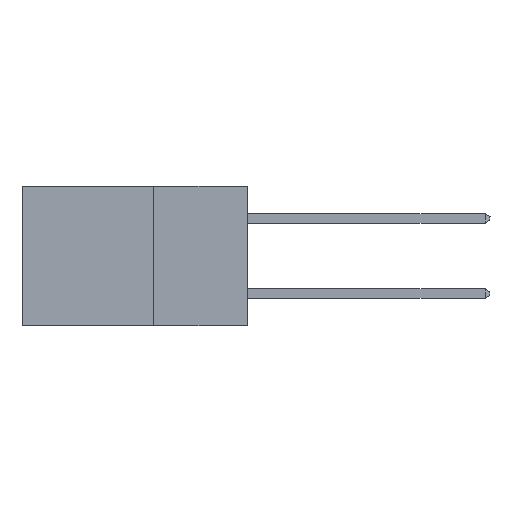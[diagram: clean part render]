
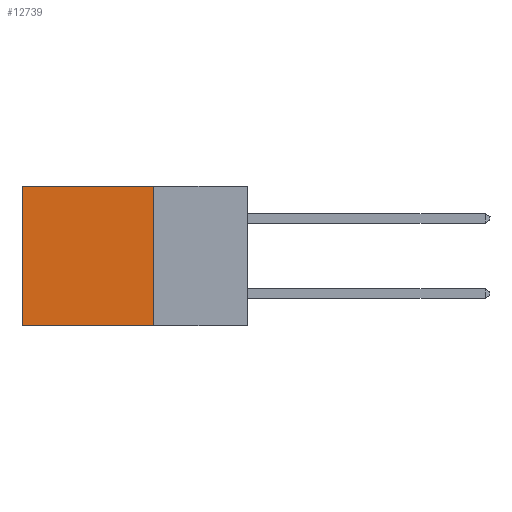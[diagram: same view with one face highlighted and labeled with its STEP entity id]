
A CAD part, left-side view. The second image highlights one B-rep face of the part: STEP entity #12739.
In plain terms, the highlighted planar face has unit normal (-1, 0, 0).
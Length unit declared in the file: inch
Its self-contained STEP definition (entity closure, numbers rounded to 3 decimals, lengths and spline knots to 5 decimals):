
#1129 = LINE ( 'NONE', #12004, #6805 ) ;
#2747 = CARTESIAN_POINT ( 'NONE',  ( 0.298, 0.25, -0.37 ) ) ;
#2850 = CARTESIAN_POINT ( 'NONE',  ( 0.298, 0.25, 0. ) ) ;
#3211 = LINE ( 'NONE', #12573, #20310 ) ;
#3948 = VECTOR ( 'NONE', #9587, 39.37008 ) ;
#4928 = DIRECTION ( 'NONE',  ( 0., 0., -1. ) ) ;
#5173 = VERTEX_POINT ( 'NONE', #20857 ) ;
#6610 = CARTESIAN_POINT ( 'NONE',  ( 0.298, 0.25, 0. ) ) ;
#6683 = DIRECTION ( 'NONE',  ( 1., 0., 0. ) ) ;
#6805 = VECTOR ( 'NONE', #4928, 39.37008 ) ;
#7255 = VERTEX_POINT ( 'NONE', #2850 ) ;
#7621 = EDGE_CURVE ( 'NONE', #7255, #5173, #3211, .T. ) ;
#7803 = FACE_OUTER_BOUND ( 'NONE', #18617, .T. ) ;
#9323 = EDGE_CURVE ( 'NONE', #5173, #23420, #1129, .T. ) ;
#9587 = DIRECTION ( 'NONE',  ( 0., 1., 0. ) ) ;
#10266 = DIRECTION ( 'NONE',  ( 0., 0., -1. ) ) ;
#10966 = ORIENTED_EDGE ( 'NONE', *, *, #9323, .T. ) ;
#11480 = VECTOR ( 'NONE', #19633, 39.37008 ) ;
#12004 = CARTESIAN_POINT ( 'NONE',  ( 0.298, 0.6, 0. ) ) ;
#12305 = CARTESIAN_POINT ( 'NONE',  ( 0.298, 0.25, 0. ) ) ;
#12573 = CARTESIAN_POINT ( 'NONE',  ( 0.298, 0.25, 0. ) ) ;
#12739 = ADVANCED_FACE ( 'NONE', ( #7803 ), #17516, .F. ) ;
#14529 = ORIENTED_EDGE ( 'NONE', *, *, #22888, .F. ) ;
#15287 = CARTESIAN_POINT ( 'NONE',  ( 0.298, 0.6, -0.37 ) ) ;
#16103 = ORIENTED_EDGE ( 'NONE', *, *, #18044, .F. ) ;
#16333 = LINE ( 'NONE', #12305, #11480 ) ;
#16691 = VERTEX_POINT ( 'NONE', #2747 ) ;
#16697 = ORIENTED_EDGE ( 'NONE', *, *, #7621, .T. ) ;
#17516 = PLANE ( 'NONE',  #18256 ) ;
#18044 = EDGE_CURVE ( 'NONE', #7255, #16691, #16333, .T. ) ;
#18256 = AXIS2_PLACEMENT_3D ( 'NONE', #6610, #6683, #10266 ) ;
#18617 = EDGE_LOOP ( 'NONE', ( #10966, #14529, #16103, #16697 ) ) ;
#18750 = CARTESIAN_POINT ( 'NONE',  ( 0.298, 0.25, -0.37 ) ) ;
#19633 = DIRECTION ( 'NONE',  ( 0., 0., -1. ) ) ;
#19653 = DIRECTION ( 'NONE',  ( 0., 1., 0. ) ) ;
#20225 = LINE ( 'NONE', #18750, #3948 ) ;
#20310 = VECTOR ( 'NONE', #19653, 39.37008 ) ;
#20857 = CARTESIAN_POINT ( 'NONE',  ( 0.298, 0.6, 0. ) ) ;
#22888 = EDGE_CURVE ( 'NONE', #16691, #23420, #20225, .T. ) ;
#23420 = VERTEX_POINT ( 'NONE', #15287 ) ;
